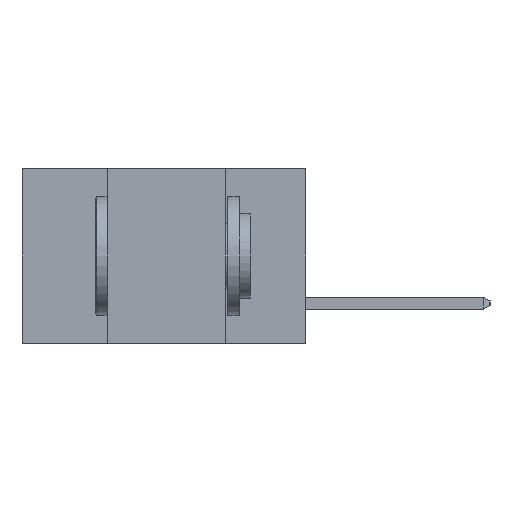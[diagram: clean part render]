
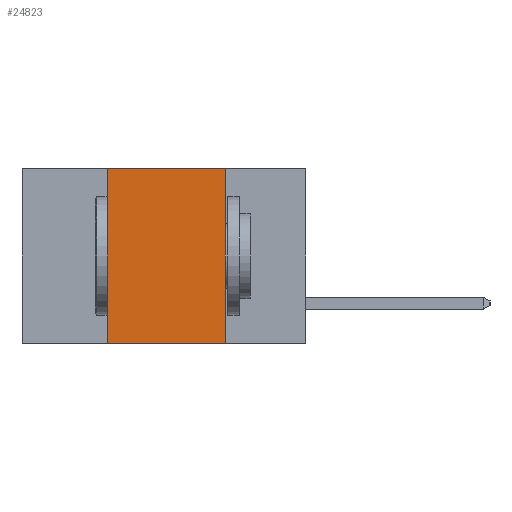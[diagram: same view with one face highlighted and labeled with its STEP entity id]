
A CAD part, left-side view. The second image highlights one B-rep face of the part: STEP entity #24823.
In plain terms, the highlighted planar face has unit normal (-1, 0, 0).
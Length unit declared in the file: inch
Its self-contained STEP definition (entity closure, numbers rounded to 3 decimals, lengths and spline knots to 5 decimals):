
#942 = LINE ( 'NONE', #25056, #7577 ) ;
#4129 = CARTESIAN_POINT ( 'NONE',  ( 0., 0.42, 0. ) ) ;
#4585 = CARTESIAN_POINT ( 'NONE',  ( 0., 0.42, -0.37 ) ) ;
#5740 = CARTESIAN_POINT ( 'NONE',  ( 0., 0.17, -0.37 ) ) ;
#6077 = LINE ( 'NONE', #19564, #11880 ) ;
#6612 = DIRECTION ( 'NONE',  ( 0., 0., 1. ) ) ;
#7486 = ORIENTED_EDGE ( 'NONE', *, *, #28706, .F. ) ;
#7577 = VECTOR ( 'NONE', #29786, 39.37008 ) ;
#7627 = LINE ( 'NONE', #29532, #26118 ) ;
#8819 = EDGE_CURVE ( 'NONE', #24553, #18022, #7627, .T. ) ;
#9303 = ORIENTED_EDGE ( 'NONE', *, *, #21293, .F. ) ;
#10467 = EDGE_CURVE ( 'NONE', #24553, #25251, #23769, .T. ) ;
#10974 = VECTOR ( 'NONE', #6612, 39.37008 ) ;
#10979 = DIRECTION ( 'NONE',  ( 1., 0., 0. ) ) ;
#11352 = ORIENTED_EDGE ( 'NONE', *, *, #10467, .F. ) ;
#11880 = VECTOR ( 'NONE', #26702, 39.37008 ) ;
#11975 = AXIS2_PLACEMENT_3D ( 'NONE', #18185, #10979, #27722 ) ;
#12833 = DIRECTION ( 'NONE',  ( 0., -1., 0. ) ) ;
#13155 = ORIENTED_EDGE ( 'NONE', *, *, #8819, .T. ) ;
#14831 = CARTESIAN_POINT ( 'NONE',  ( 0., 0.17, 0. ) ) ;
#18022 = VERTEX_POINT ( 'NONE', #5740 ) ;
#18185 = CARTESIAN_POINT ( 'NONE',  ( 0., 0.6, 0. ) ) ;
#19564 = CARTESIAN_POINT ( 'NONE',  ( 0., 0.6, 0. ) ) ;
#21293 = EDGE_CURVE ( 'NONE', #25251, #25916, #6077, .T. ) ;
#23769 = LINE ( 'NONE', #4129, #10974 ) ;
#24468 = FACE_OUTER_BOUND ( 'NONE', #26860, .T. ) ;
#24553 = VERTEX_POINT ( 'NONE', #4585 ) ;
#24823 = ADVANCED_FACE ( 'NONE', ( #24468 ), #25344, .F. ) ;
#25056 = CARTESIAN_POINT ( 'NONE',  ( 0., 0.17, 0. ) ) ;
#25251 = VERTEX_POINT ( 'NONE', #26761 ) ;
#25344 = PLANE ( 'NONE',  #11975 ) ;
#25916 = VERTEX_POINT ( 'NONE', #14831 ) ;
#26118 = VECTOR ( 'NONE', #12833, 39.37008 ) ;
#26702 = DIRECTION ( 'NONE',  ( 0., -1., 0. ) ) ;
#26761 = CARTESIAN_POINT ( 'NONE',  ( 0., 0.42, 0. ) ) ;
#26860 = EDGE_LOOP ( 'NONE', ( #7486, #9303, #11352, #13155 ) ) ;
#27722 = DIRECTION ( 'NONE',  ( 0., 0., -1. ) ) ;
#28706 = EDGE_CURVE ( 'NONE', #25916, #18022, #942, .T. ) ;
#29532 = CARTESIAN_POINT ( 'NONE',  ( 0., 0.6, -0.37 ) ) ;
#29786 = DIRECTION ( 'NONE',  ( 0., 0., -1. ) ) ;
